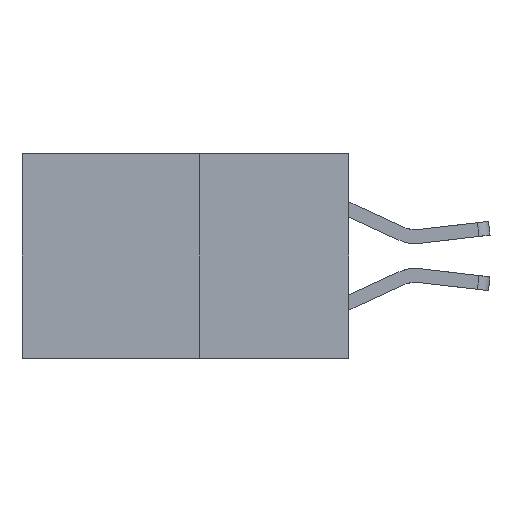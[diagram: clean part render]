
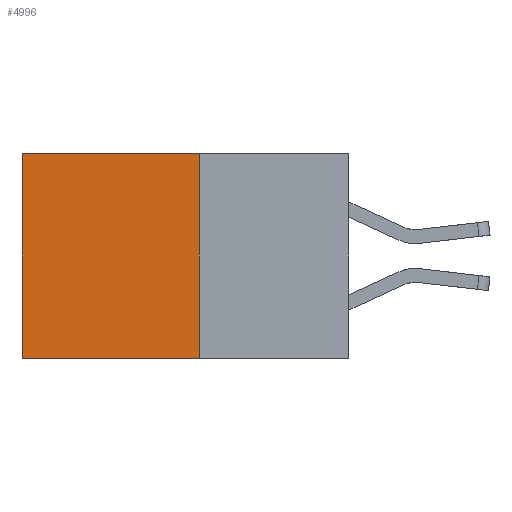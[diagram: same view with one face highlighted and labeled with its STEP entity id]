
A CAD part, left-side view. The second image highlights one B-rep face of the part: STEP entity #4996.
In plain terms, the highlighted planar face has unit normal (-1, 0, 0).
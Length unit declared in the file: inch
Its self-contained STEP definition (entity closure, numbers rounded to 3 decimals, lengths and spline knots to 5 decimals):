
#83 = CARTESIAN_POINT ( 'NONE',  ( 0.277, 0.27, 0. ) ) ;
#242 = FACE_OUTER_BOUND ( 'NONE', #6948, .T. ) ;
#390 = EDGE_CURVE ( 'NONE', #6562, #7542, #9171, .T. ) ;
#764 = CARTESIAN_POINT ( 'NONE',  ( 0.277, 0.27, 0. ) ) ;
#1035 = AXIS2_PLACEMENT_3D ( 'NONE', #1513, #8707, #2965 ) ;
#1513 = CARTESIAN_POINT ( 'NONE',  ( 0.277, 0.27, -0.37 ) ) ;
#1770 = DIRECTION ( 'NONE',  ( 0., 0., -1. ) ) ;
#1997 = DIRECTION ( 'NONE',  ( 0., 1., 0. ) ) ;
#2226 = PLANE ( 'NONE',  #1035 ) ;
#2965 = DIRECTION ( 'NONE',  ( 0., 0., -1. ) ) ;
#3100 = CARTESIAN_POINT ( 'NONE',  ( 0.277, 0.27, -0.37 ) ) ;
#3113 = ORIENTED_EDGE ( 'NONE', *, *, #4484, .F. ) ;
#3145 = DIRECTION ( 'NONE',  ( 0., 0., -1. ) ) ;
#3213 = CARTESIAN_POINT ( 'NONE',  ( 0.277, 0.59, -0.37 ) ) ;
#3328 = ORIENTED_EDGE ( 'NONE', *, *, #390, .T. ) ;
#3908 = VERTEX_POINT ( 'NONE', #3213 ) ;
#4113 = ORIENTED_EDGE ( 'NONE', *, *, #5693, .F. ) ;
#4484 = EDGE_CURVE ( 'NONE', #8957, #3908, #6298, .T. ) ;
#4583 = DIRECTION ( 'NONE',  ( 0., 1., 0. ) ) ;
#4981 = LINE ( 'NONE', #5433, #6219 ) ;
#4996 = ADVANCED_FACE ( 'NONE', ( #242 ), #2226, .F. ) ;
#5402 = VECTOR ( 'NONE', #3145, 39.37008 ) ;
#5433 = CARTESIAN_POINT ( 'NONE',  ( 0.277, 0.59, -0.37 ) ) ;
#5693 = EDGE_CURVE ( 'NONE', #6562, #8957, #9232, .T. ) ;
#5708 = CARTESIAN_POINT ( 'NONE',  ( 0.277, 0.27, -0.37 ) ) ;
#6076 = VECTOR ( 'NONE', #4583, 39.37008 ) ;
#6219 = VECTOR ( 'NONE', #1770, 39.37008 ) ;
#6298 = LINE ( 'NONE', #3100, #6076 ) ;
#6562 = VERTEX_POINT ( 'NONE', #83 ) ;
#6765 = CARTESIAN_POINT ( 'NONE',  ( 0.277, 0.27, -0.37 ) ) ;
#6948 = EDGE_LOOP ( 'NONE', ( #9187, #3113, #4113, #3328 ) ) ;
#7029 = VECTOR ( 'NONE', #1997, 39.37008 ) ;
#7542 = VERTEX_POINT ( 'NONE', #8451 ) ;
#8011 = EDGE_CURVE ( 'NONE', #7542, #3908, #4981, .T. ) ;
#8451 = CARTESIAN_POINT ( 'NONE',  ( 0.277, 0.59, 0. ) ) ;
#8707 = DIRECTION ( 'NONE',  ( 1., 0., 0. ) ) ;
#8957 = VERTEX_POINT ( 'NONE', #5708 ) ;
#9171 = LINE ( 'NONE', #764, #7029 ) ;
#9187 = ORIENTED_EDGE ( 'NONE', *, *, #8011, .T. ) ;
#9232 = LINE ( 'NONE', #6765, #5402 ) ;
